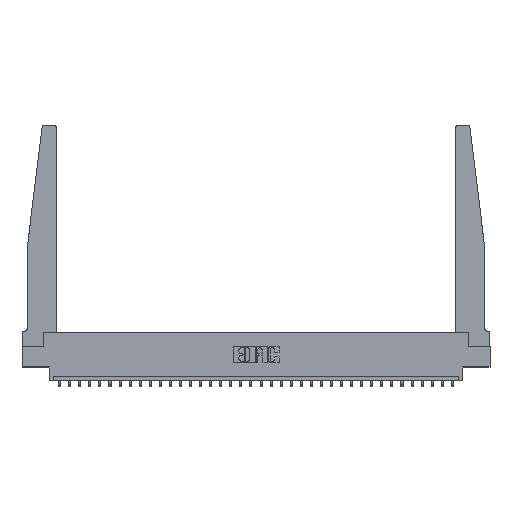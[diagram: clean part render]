
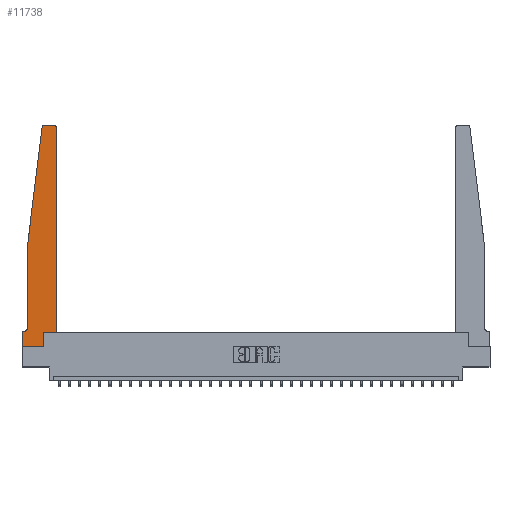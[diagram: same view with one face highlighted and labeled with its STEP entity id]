
A CAD part, top view. The second image highlights one B-rep face of the part: STEP entity #11738.
In plain terms, the highlighted planar face has unit normal (0, 0, 1).
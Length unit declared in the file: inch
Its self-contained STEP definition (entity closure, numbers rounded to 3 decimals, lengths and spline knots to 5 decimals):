
#544 = CIRCLE ( 'NONE', #2033, 0.03 ) ;
#561 = CARTESIAN_POINT ( 'NONE',  ( 0.425, 0.18, 0.37 ) ) ;
#758 = CARTESIAN_POINT ( 'NONE',  ( 0.2605, 0.18, 0.37 ) ) ;
#867 = VERTEX_POINT ( 'NONE', #20350 ) ;
#906 = DIRECTION ( 'NONE',  ( 0., 1., 0. ) ) ;
#1419 = VERTEX_POINT ( 'NONE', #16720 ) ;
#1645 = VERTEX_POINT ( 'NONE', #27503 ) ;
#2033 = AXIS2_PLACEMENT_3D ( 'NONE', #8894, #23082, #12119 ) ;
#2382 = VERTEX_POINT ( 'NONE', #2792 ) ;
#2748 = CARTESIAN_POINT ( 'NONE',  ( 0.015, 0.2375, 0.37 ) ) ;
#2792 = CARTESIAN_POINT ( 'NONE',  ( 0., 0., 0.37 ) ) ;
#3083 = CARTESIAN_POINT ( 'NONE',  ( 0.065, 0.1875, 0.37 ) ) ;
#3159 = LINE ( 'NONE', #5793, #9725 ) ;
#3235 = ORIENTED_EDGE ( 'NONE', *, *, #26477, .T. ) ;
#3897 = DIRECTION ( 'NONE',  ( 0., -1., 0. ) ) ;
#4105 = CARTESIAN_POINT ( 'NONE',  ( 0.2605, 0., 0.37 ) ) ;
#4372 = ORIENTED_EDGE ( 'NONE', *, *, #28183, .T. ) ;
#4792 = VERTEX_POINT ( 'NONE', #26321 ) ;
#5096 = DIRECTION ( 'NONE',  ( -1., 0., 0. ) ) ;
#5323 = AXIS2_PLACEMENT_3D ( 'NONE', #2748, #23449, #5096 ) ;
#5566 = VERTEX_POINT ( 'NONE', #11740 ) ;
#5793 = CARTESIAN_POINT ( 'NONE',  ( 0.065, 1.25, 0.37 ) ) ;
#5906 = VECTOR ( 'NONE', #7278, 39.37008 ) ;
#6011 = VERTEX_POINT ( 'NONE', #8190 ) ;
#6027 = EDGE_CURVE ( 'NONE', #867, #5566, #22265, .T. ) ;
#6077 = DIRECTION ( 'NONE',  ( 1., 0., 0. ) ) ;
#7278 = DIRECTION ( 'NONE',  ( -1., 0., 0. ) ) ;
#7469 = VECTOR ( 'NONE', #27497, 39.37008 ) ;
#8190 = CARTESIAN_POINT ( 'NONE',  ( 0.2605, 0.18, 0.37 ) ) ;
#8650 = DIRECTION ( 'NONE',  ( 1., 0., 0. ) ) ;
#8691 = LINE ( 'NONE', #22278, #23637 ) ;
#8894 = CARTESIAN_POINT ( 'NONE',  ( 0.27653, 2.72, 0.37 ) ) ;
#8946 = VECTOR ( 'NONE', #18106, 39.37008 ) ;
#9254 = EDGE_CURVE ( 'NONE', #10058, #6011, #22199, .T. ) ;
#9527 = EDGE_CURVE ( 'NONE', #2382, #10058, #28787, .T. ) ;
#9725 = VECTOR ( 'NONE', #22449, 39.37008 ) ;
#9864 = ORIENTED_EDGE ( 'NONE', *, *, #25051, .T. ) ;
#9899 = AXIS2_PLACEMENT_3D ( 'NONE', #29250, #22424, #6077 ) ;
#10058 = VERTEX_POINT ( 'NONE', #4105 ) ;
#10390 = ORIENTED_EDGE ( 'NONE', *, *, #24234, .T. ) ;
#10706 = VERTEX_POINT ( 'NONE', #24051 ) ;
#11135 = CARTESIAN_POINT ( 'NONE',  ( 0.425, 0.18, 0.37 ) ) ;
#11738 = ADVANCED_FACE ( 'NONE', ( #20097 ), #17357, .T. ) ;
#11740 = CARTESIAN_POINT ( 'NONE',  ( 0.395, 2.75, 0.37 ) ) ;
#12119 = DIRECTION ( 'NONE',  ( 1., 0., 0. ) ) ;
#12755 = CARTESIAN_POINT ( 'NONE',  ( 0.425, 0.18, 0.37 ) ) ;
#12943 = LINE ( 'NONE', #28436, #5906 ) ;
#13812 = VERTEX_POINT ( 'NONE', #26840 ) ;
#13920 = EDGE_CURVE ( 'NONE', #5566, #10706, #12943, .T. ) ;
#14018 = DIRECTION ( 'NONE',  ( 1., 0., 0. ) ) ;
#14583 = CARTESIAN_POINT ( 'NONE',  ( 0., 0., 0.37 ) ) ;
#14934 = DIRECTION ( 'NONE',  ( 0., 1., 0. ) ) ;
#15134 = ORIENTED_EDGE ( 'NONE', *, *, #9527, .T. ) ;
#15873 = AXIS2_PLACEMENT_3D ( 'NONE', #17751, #17908, #8650 ) ;
#16154 = EDGE_CURVE ( 'NONE', #27246, #2382, #22740, .T. ) ;
#16720 = CARTESIAN_POINT ( 'NONE',  ( 0.065, 1.25, 0.37 ) ) ;
#17357 = PLANE ( 'NONE',  #9899 ) ;
#17741 = EDGE_CURVE ( 'NONE', #10706, #13812, #544, .T. ) ;
#17751 = CARTESIAN_POINT ( 'NONE',  ( 0.395, 2.72, 0.37 ) ) ;
#17908 = DIRECTION ( 'NONE',  ( 0., 0., 1. ) ) ;
#17993 = EDGE_CURVE ( 'NONE', #6011, #26996, #18078, .T. ) ;
#18078 = LINE ( 'NONE', #11135, #7469 ) ;
#18106 = DIRECTION ( 'NONE',  ( 0., -1., 0. ) ) ;
#20097 = FACE_OUTER_BOUND ( 'NONE', #24939, .T. ) ;
#20350 = CARTESIAN_POINT ( 'NONE',  ( 0.425, 2.72, 0.37 ) ) ;
#21023 = ORIENTED_EDGE ( 'NONE', *, *, #13920, .T. ) ;
#21072 = CIRCLE ( 'NONE', #5323, 0.05 ) ;
#21602 = ORIENTED_EDGE ( 'NONE', *, *, #16154, .T. ) ;
#22047 = ORIENTED_EDGE ( 'NONE', *, *, #9254, .T. ) ;
#22199 = LINE ( 'NONE', #758, #27123 ) ;
#22265 = CIRCLE ( 'NONE', #15873, 0.03 ) ;
#22278 = CARTESIAN_POINT ( 'NONE',  ( 0.065, 1.25, 0.37 ) ) ;
#22424 = DIRECTION ( 'NONE',  ( 0., 0., 1. ) ) ;
#22449 = DIRECTION ( 'NONE',  ( -0.122, -0.992, 0. ) ) ;
#22740 = LINE ( 'NONE', #27065, #8946 ) ;
#23082 = DIRECTION ( 'NONE',  ( 0., 0., 1. ) ) ;
#23449 = DIRECTION ( 'NONE',  ( 0., 0., -1. ) ) ;
#23637 = VECTOR ( 'NONE', #3897, 39.37008 ) ;
#24051 = CARTESIAN_POINT ( 'NONE',  ( 0.27653, 2.75, 0.37 ) ) ;
#24082 = ORIENTED_EDGE ( 'NONE', *, *, #17993, .T. ) ;
#24159 = ORIENTED_EDGE ( 'NONE', *, *, #28804, .T. ) ;
#24234 = EDGE_CURVE ( 'NONE', #1645, #27246, #24393, .T. ) ;
#24393 = LINE ( 'NONE', #3083, #27867 ) ;
#24939 = EDGE_LOOP ( 'NONE', ( #21023, #28788, #9864, #24159, #3235, #10390, #21602, #15134, #22047, #24082, #4372, #25916 ) ) ;
#25051 = EDGE_CURVE ( 'NONE', #13812, #1419, #3159, .T. ) ;
#25850 = CARTESIAN_POINT ( 'NONE',  ( 0., 0.1875, 0.37 ) ) ;
#25916 = ORIENTED_EDGE ( 'NONE', *, *, #6027, .T. ) ;
#26249 = DIRECTION ( 'NONE',  ( -1., 0., 0. ) ) ;
#26321 = CARTESIAN_POINT ( 'NONE',  ( 0.065, 0.2375, 0.37 ) ) ;
#26477 = EDGE_CURVE ( 'NONE', #4792, #1645, #21072, .T. ) ;
#26840 = CARTESIAN_POINT ( 'NONE',  ( 0.24675, 2.72367, 0.37 ) ) ;
#26996 = VERTEX_POINT ( 'NONE', #561 ) ;
#27065 = CARTESIAN_POINT ( 'NONE',  ( 0., 0., 0.37 ) ) ;
#27123 = VECTOR ( 'NONE', #906, 39.37008 ) ;
#27246 = VERTEX_POINT ( 'NONE', #25850 ) ;
#27497 = DIRECTION ( 'NONE',  ( 1., 0., 0. ) ) ;
#27503 = CARTESIAN_POINT ( 'NONE',  ( 0.015, 0.1875, 0.37 ) ) ;
#27867 = VECTOR ( 'NONE', #26249, 39.37008 ) ;
#28183 = EDGE_CURVE ( 'NONE', #26996, #867, #28971, .T. ) ;
#28187 = VECTOR ( 'NONE', #14018, 39.37008 ) ;
#28436 = CARTESIAN_POINT ( 'NONE',  ( 0.25, 2.75, 0.37 ) ) ;
#28787 = LINE ( 'NONE', #14583, #28187 ) ;
#28788 = ORIENTED_EDGE ( 'NONE', *, *, #17741, .T. ) ;
#28804 = EDGE_CURVE ( 'NONE', #1419, #4792, #8691, .T. ) ;
#28971 = LINE ( 'NONE', #12755, #29060 ) ;
#29060 = VECTOR ( 'NONE', #14934, 39.37008 ) ;
#29250 = CARTESIAN_POINT ( 'NONE',  ( 0., 0.1875, 0.37 ) ) ;
